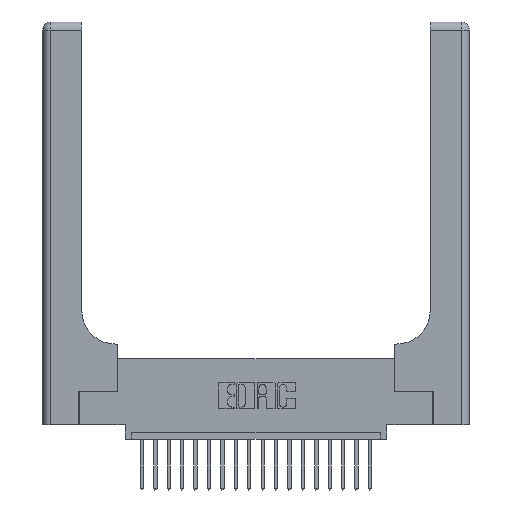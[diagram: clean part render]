
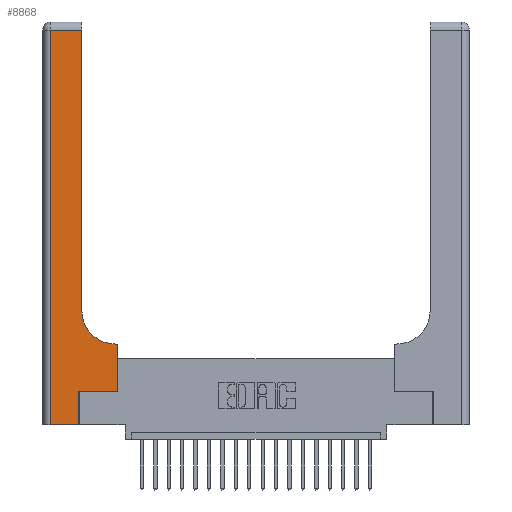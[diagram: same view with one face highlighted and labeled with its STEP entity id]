
A CAD part, top view. The second image highlights one B-rep face of the part: STEP entity #8868.
In plain terms, the highlighted planar face has unit normal (0, 0, 1).
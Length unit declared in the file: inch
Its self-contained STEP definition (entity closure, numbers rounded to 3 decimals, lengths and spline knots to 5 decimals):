
#11 = VERTEX_POINT ( 'NONE', #18635 ) ;
#336 = ORIENTED_EDGE ( 'NONE', *, *, #20156, .T. ) ;
#579 = EDGE_CURVE ( 'NONE', #16200, #7667, #754, .T. ) ;
#754 = LINE ( 'NONE', #10641, #7925 ) ;
#877 = LINE ( 'NONE', #4805, #21427 ) ;
#1104 = DIRECTION ( 'NONE',  ( 0., 0., -1. ) ) ;
#1211 = AXIS2_PLACEMENT_3D ( 'NONE', #6716, #8631, #8552 ) ;
#1233 = DIRECTION ( 'NONE',  ( 1., 0., 0. ) ) ;
#1776 = EDGE_CURVE ( 'NONE', #5346, #11227, #16120, .T. ) ;
#2390 = CARTESIAN_POINT ( 'NONE',  ( 0.2915, 2.94, 0.37 ) ) ;
#2476 = DIRECTION ( 'NONE',  ( -1., 0., 0. ) ) ;
#2741 = EDGE_CURVE ( 'NONE', #11, #5346, #18514, .T. ) ;
#2774 = CARTESIAN_POINT ( 'NONE',  ( 0.06, 3., 0.37 ) ) ;
#2911 = CARTESIAN_POINT ( 'NONE',  ( 0.2915, 3., 0.37 ) ) ;
#3621 = ORIENTED_EDGE ( 'NONE', *, *, #13819, .T. ) ;
#4369 = ORIENTED_EDGE ( 'NONE', *, *, #20027, .T. ) ;
#4587 = EDGE_CURVE ( 'NONE', #18744, #11, #6692, .T. ) ;
#4805 = CARTESIAN_POINT ( 'NONE',  ( 0.269, 0.25, 0.37 ) ) ;
#4880 = LINE ( 'NONE', #17595, #5187 ) ;
#5187 = VECTOR ( 'NONE', #2476, 39.37008 ) ;
#5346 = VERTEX_POINT ( 'NONE', #9018 ) ;
#5416 = LINE ( 'NONE', #2911, #9898 ) ;
#6186 = CARTESIAN_POINT ( 'NONE',  ( 0.5585, 0.25, 0.37 ) ) ;
#6467 = VECTOR ( 'NONE', #8481, 39.37008 ) ;
#6489 = CARTESIAN_POINT ( 'NONE',  ( 0.2915, 0.85, 0.37 ) ) ;
#6542 = DIRECTION ( 'NONE',  ( 1., 0., 0. ) ) ;
#6692 = LINE ( 'NONE', #15452, #21923 ) ;
#6716 = CARTESIAN_POINT ( 'NONE',  ( 0., 3., 0.37 ) ) ;
#7196 = VERTEX_POINT ( 'NONE', #16358 ) ;
#7667 = VERTEX_POINT ( 'NONE', #12248 ) ;
#7925 = VECTOR ( 'NONE', #1233, 39.37008 ) ;
#8036 = LINE ( 'NONE', #17044, #6467 ) ;
#8081 = ORIENTED_EDGE ( 'NONE', *, *, #1776, .T. ) ;
#8481 = DIRECTION ( 'NONE',  ( 0., 1., 0. ) ) ;
#8552 = DIRECTION ( 'NONE',  ( -1., 0., 0. ) ) ;
#8631 = DIRECTION ( 'NONE',  ( 0., 0., -1. ) ) ;
#8670 = EDGE_CURVE ( 'NONE', #20731, #21028, #4880, .T. ) ;
#8804 = EDGE_CURVE ( 'NONE', #21028, #16200, #9928, .T. ) ;
#8868 = ADVANCED_FACE ( 'NONE', ( #11549 ), #18793, .F. ) ;
#8898 = ORIENTED_EDGE ( 'NONE', *, *, #579, .T. ) ;
#9018 = CARTESIAN_POINT ( 'NONE',  ( 0.5415, 0.6, 0.37 ) ) ;
#9898 = VECTOR ( 'NONE', #11705, 39.37008 ) ;
#9928 = LINE ( 'NONE', #2774, #13693 ) ;
#10010 = DIRECTION ( 'NONE',  ( 1., 0., 0. ) ) ;
#10389 = AXIS2_PLACEMENT_3D ( 'NONE', #16704, #1104, #6542 ) ;
#10641 = CARTESIAN_POINT ( 'NONE',  ( 0., 0., 0.37 ) ) ;
#11227 = VERTEX_POINT ( 'NONE', #6489 ) ;
#11549 = FACE_OUTER_BOUND ( 'NONE', #19775, .T. ) ;
#11705 = DIRECTION ( 'NONE',  ( 0., 1., 0. ) ) ;
#12248 = CARTESIAN_POINT ( 'NONE',  ( 0.269, 0., 0.37 ) ) ;
#12944 = CARTESIAN_POINT ( 'NONE',  ( 0.06, 0., 0.37 ) ) ;
#13693 = VECTOR ( 'NONE', #19933, 39.37008 ) ;
#13819 = EDGE_CURVE ( 'NONE', #7196, #18744, #877, .T. ) ;
#14448 = ORIENTED_EDGE ( 'NONE', *, *, #2741, .T. ) ;
#15452 = CARTESIAN_POINT ( 'NONE',  ( 0.5585, 0.25, 0.37 ) ) ;
#16120 = CIRCLE ( 'NONE', #10389, 0.25 ) ;
#16200 = VERTEX_POINT ( 'NONE', #12944 ) ;
#16286 = DIRECTION ( 'NONE',  ( -1., 0., 0. ) ) ;
#16358 = CARTESIAN_POINT ( 'NONE',  ( 0.269, 0.25, 0.37 ) ) ;
#16704 = CARTESIAN_POINT ( 'NONE',  ( 0.5415, 0.85, 0.37 ) ) ;
#17044 = CARTESIAN_POINT ( 'NONE',  ( 0.269, 0., 0.37 ) ) ;
#17246 = DIRECTION ( 'NONE',  ( 0., 1., 0. ) ) ;
#17595 = CARTESIAN_POINT ( 'NONE',  ( 0., 2.94, 0.37 ) ) ;
#17915 = ORIENTED_EDGE ( 'NONE', *, *, #8670, .T. ) ;
#17971 = VECTOR ( 'NONE', #16286, 39.37008 ) ;
#18514 = LINE ( 'NONE', #21200, #17971 ) ;
#18635 = CARTESIAN_POINT ( 'NONE',  ( 0.5585, 0.6, 0.37 ) ) ;
#18744 = VERTEX_POINT ( 'NONE', #6186 ) ;
#18793 = PLANE ( 'NONE',  #1211 ) ;
#19775 = EDGE_LOOP ( 'NONE', ( #4369, #17915, #20065, #8898, #336, #3621, #20788, #14448, #8081 ) ) ;
#19933 = DIRECTION ( 'NONE',  ( 0., -1., 0. ) ) ;
#20027 = EDGE_CURVE ( 'NONE', #11227, #20731, #5416, .T. ) ;
#20065 = ORIENTED_EDGE ( 'NONE', *, *, #8804, .T. ) ;
#20156 = EDGE_CURVE ( 'NONE', #7667, #7196, #8036, .T. ) ;
#20731 = VERTEX_POINT ( 'NONE', #2390 ) ;
#20788 = ORIENTED_EDGE ( 'NONE', *, *, #4587, .T. ) ;
#21028 = VERTEX_POINT ( 'NONE', #21569 ) ;
#21200 = CARTESIAN_POINT ( 'NONE',  ( 0.2915, 0.6, 0.37 ) ) ;
#21427 = VECTOR ( 'NONE', #10010, 39.37008 ) ;
#21569 = CARTESIAN_POINT ( 'NONE',  ( 0.06, 2.94, 0.37 ) ) ;
#21923 = VECTOR ( 'NONE', #17246, 39.37008 ) ;
